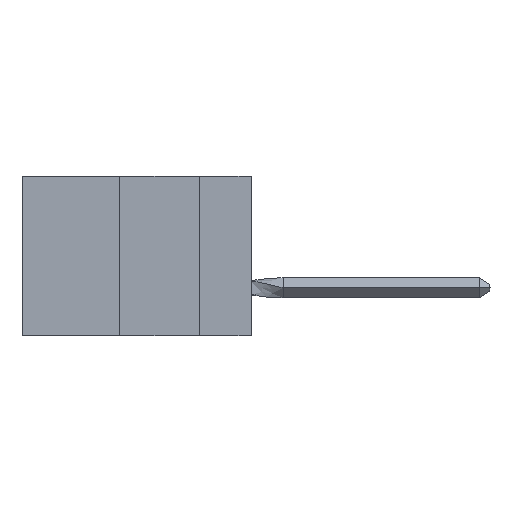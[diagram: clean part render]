
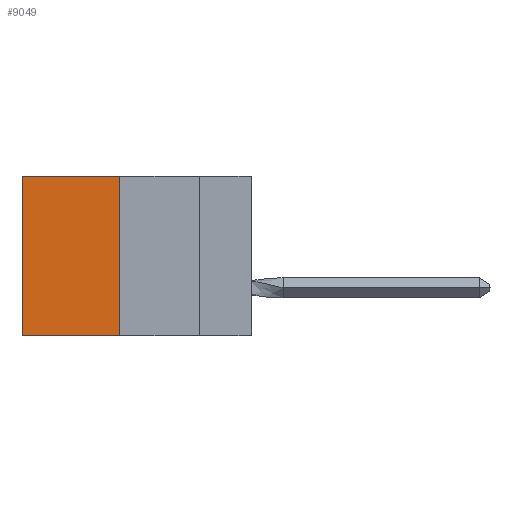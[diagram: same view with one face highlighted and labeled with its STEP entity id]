
A CAD part, left-side view. The second image highlights one B-rep face of the part: STEP entity #9049.
In plain terms, the highlighted planar face has unit normal (-1, 0, 0).
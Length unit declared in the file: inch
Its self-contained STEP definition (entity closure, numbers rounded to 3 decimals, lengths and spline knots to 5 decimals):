
#895 = DIRECTION ( 'NONE',  ( 0., 1., 0. ) ) ;
#3363 = CARTESIAN_POINT ( 'NONE',  ( 0.305, 0.72, -0.5 ) ) ;
#4557 = CARTESIAN_POINT ( 'NONE',  ( 0.305, 0.413, -0.5 ) ) ;
#4920 = ORIENTED_EDGE ( 'NONE', *, *, #7907, .F. ) ;
#5276 = LINE ( 'NONE', #22995, #22315 ) ;
#5286 = DIRECTION ( 'NONE',  ( 1., 0., 0. ) ) ;
#5295 = DIRECTION ( 'NONE',  ( 0., 0., -1. ) ) ;
#6458 = LINE ( 'NONE', #11883, #9947 ) ;
#6509 = LINE ( 'NONE', #3363, #18644 ) ;
#7552 = ORIENTED_EDGE ( 'NONE', *, *, #14167, .T. ) ;
#7838 = CARTESIAN_POINT ( 'NONE',  ( 0.305, 0.72, 0. ) ) ;
#7872 = ORIENTED_EDGE ( 'NONE', *, *, #14447, .T. ) ;
#7899 = EDGE_CURVE ( 'NONE', #14193, #10745, #5276, .T. ) ;
#7907 = EDGE_CURVE ( 'NONE', #10745, #17454, #6458, .T. ) ;
#7981 = CARTESIAN_POINT ( 'NONE',  ( 0.305, 0.413, 0. ) ) ;
#9049 = ADVANCED_FACE ( 'NONE', ( #11875 ), #14431, .F. ) ;
#9090 = ORIENTED_EDGE ( 'NONE', *, *, #7899, .F. ) ;
#9947 = VECTOR ( 'NONE', #895, 39.37008 ) ;
#10495 = CARTESIAN_POINT ( 'NONE',  ( 0.305, 0.72, -0.5 ) ) ;
#10745 = VERTEX_POINT ( 'NONE', #4557 ) ;
#11875 = FACE_OUTER_BOUND ( 'NONE', #19779, .T. ) ;
#11883 = CARTESIAN_POINT ( 'NONE',  ( 0.305, 0.413, -0.5 ) ) ;
#11976 = DIRECTION ( 'NONE',  ( 0., 0., -1. ) ) ;
#12010 = VECTOR ( 'NONE', #17263, 39.37008 ) ;
#13165 = LINE ( 'NONE', #7981, #12010 ) ;
#13256 = CARTESIAN_POINT ( 'NONE',  ( 0.305, 0.413, 0. ) ) ;
#13706 = VERTEX_POINT ( 'NONE', #7838 ) ;
#14167 = EDGE_CURVE ( 'NONE', #13706, #17454, #6509, .T. ) ;
#14193 = VERTEX_POINT ( 'NONE', #13256 ) ;
#14431 = PLANE ( 'NONE',  #21534 ) ;
#14447 = EDGE_CURVE ( 'NONE', #14193, #13706, #13165, .T. ) ;
#17263 = DIRECTION ( 'NONE',  ( 0., 1., 0. ) ) ;
#17454 = VERTEX_POINT ( 'NONE', #10495 ) ;
#18644 = VECTOR ( 'NONE', #5295, 39.37008 ) ;
#19779 = EDGE_LOOP ( 'NONE', ( #7552, #4920, #9090, #7872 ) ) ;
#20227 = DIRECTION ( 'NONE',  ( 0., 0., -1. ) ) ;
#21534 = AXIS2_PLACEMENT_3D ( 'NONE', #22055, #5286, #20227 ) ;
#22055 = CARTESIAN_POINT ( 'NONE',  ( 0.305, 0.413, -0.5 ) ) ;
#22315 = VECTOR ( 'NONE', #11976, 39.37008 ) ;
#22995 = CARTESIAN_POINT ( 'NONE',  ( 0.305, 0.413, -0.5 ) ) ;
